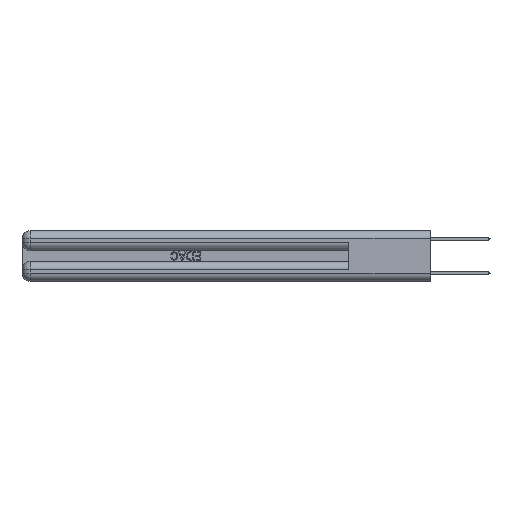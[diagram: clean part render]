
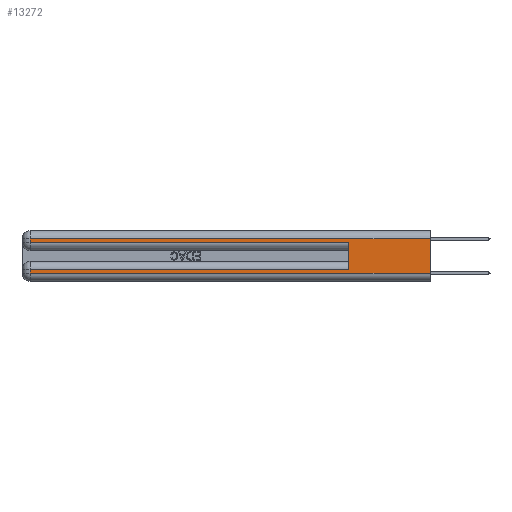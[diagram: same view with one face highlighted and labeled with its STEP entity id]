
A CAD part, left-side view. The second image highlights one B-rep face of the part: STEP entity #13272.
In plain terms, the highlighted planar face has unit normal (-1, 0, 0).
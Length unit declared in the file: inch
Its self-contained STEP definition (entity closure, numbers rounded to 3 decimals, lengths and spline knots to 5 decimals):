
#130 = CARTESIAN_POINT ( 'NONE',  ( 0., 0., 0.37 ) ) ;
#244 = DIRECTION ( 'NONE',  ( 0., 0., -1. ) ) ;
#490 = DIRECTION ( 'NONE',  ( 0., -1., 0. ) ) ;
#535 = CARTESIAN_POINT ( 'NONE',  ( 0., 0., 0.37 ) ) ;
#685 = AXIS2_PLACEMENT_3D ( 'NONE', #130, #22805, #11652 ) ;
#1635 = CARTESIAN_POINT ( 'NONE',  ( 0., 0.6, 0.085 ) ) ;
#1852 = ORIENTED_EDGE ( 'NONE', *, *, #2082, .T. ) ;
#2082 = EDGE_CURVE ( 'NONE', #6087, #33035, #23856, .T. ) ;
#2722 = CARTESIAN_POINT ( 'NONE',  ( 0., 0., 0.06 ) ) ;
#3221 = ORIENTED_EDGE ( 'NONE', *, *, #21603, .F. ) ;
#3281 = LINE ( 'NONE', #2722, #4337 ) ;
#3654 = EDGE_CURVE ( 'NONE', #15670, #11428, #26232, .T. ) ;
#4158 = CARTESIAN_POINT ( 'NONE',  ( 0., 0., 0.06 ) ) ;
#4337 = VECTOR ( 'NONE', #490, 39.37008 ) ;
#5796 = VECTOR ( 'NONE', #18809, 39.37008 ) ;
#5928 = CARTESIAN_POINT ( 'NONE',  ( 0., 2.94, 0.285 ) ) ;
#5946 = EDGE_CURVE ( 'NONE', #33035, #25880, #15562, .T. ) ;
#6087 = VERTEX_POINT ( 'NONE', #1635 ) ;
#6418 = EDGE_CURVE ( 'NONE', #6087, #16569, #23719, .T. ) ;
#6473 = CARTESIAN_POINT ( 'NONE',  ( 0., 2.94, 0.37 ) ) ;
#7280 = CARTESIAN_POINT ( 'NONE',  ( 0., 0., 0.285 ) ) ;
#7645 = ORIENTED_EDGE ( 'NONE', *, *, #17243, .T. ) ;
#8896 = VECTOR ( 'NONE', #15310, 39.37008 ) ;
#9559 = LINE ( 'NONE', #29604, #14736 ) ;
#10016 = ORIENTED_EDGE ( 'NONE', *, *, #5946, .T. ) ;
#11428 = VERTEX_POINT ( 'NONE', #5928 ) ;
#11595 = VECTOR ( 'NONE', #20779, 39.37008 ) ;
#11652 = DIRECTION ( 'NONE',  ( 0., 0., -1. ) ) ;
#12720 = DIRECTION ( 'NONE',  ( 0., 1., 0. ) ) ;
#13272 = ADVANCED_FACE ( 'NONE', ( #22987 ), #25935, .F. ) ;
#14736 = VECTOR ( 'NONE', #12720, 39.37008 ) ;
#15310 = DIRECTION ( 'NONE',  ( 0., 1., 0. ) ) ;
#15562 = LINE ( 'NONE', #6473, #11595 ) ;
#15670 = VERTEX_POINT ( 'NONE', #23554 ) ;
#15730 = CARTESIAN_POINT ( 'NONE',  ( 0., 2.94, 0.06 ) ) ;
#16569 = VERTEX_POINT ( 'NONE', #35705 ) ;
#17243 = EDGE_CURVE ( 'NONE', #25880, #35130, #3281, .T. ) ;
#17731 = VERTEX_POINT ( 'NONE', #25338 ) ;
#18809 = DIRECTION ( 'NONE',  ( 0., -1., 0. ) ) ;
#20038 = ORIENTED_EDGE ( 'NONE', *, *, #26740, .T. ) ;
#20779 = DIRECTION ( 'NONE',  ( 0., 0., -1. ) ) ;
#21052 = LINE ( 'NONE', #7280, #5796 ) ;
#21603 = EDGE_CURVE ( 'NONE', #17731, #35130, #34700, .T. ) ;
#22805 = DIRECTION ( 'NONE',  ( 1., 0., 0. ) ) ;
#22808 = ORIENTED_EDGE ( 'NONE', *, *, #27815, .T. ) ;
#22987 = FACE_OUTER_BOUND ( 'NONE', #29051, .T. ) ;
#23554 = CARTESIAN_POINT ( 'NONE',  ( 0., 2.94, 0.31 ) ) ;
#23719 = LINE ( 'NONE', #30005, #33558 ) ;
#23856 = LINE ( 'NONE', #26453, #8896 ) ;
#24526 = VECTOR ( 'NONE', #244, 39.37008 ) ;
#25186 = ORIENTED_EDGE ( 'NONE', *, *, #6418, .F. ) ;
#25338 = CARTESIAN_POINT ( 'NONE',  ( 0., 0., 0.31 ) ) ;
#25880 = VERTEX_POINT ( 'NONE', #15730 ) ;
#25935 = PLANE ( 'NONE',  #685 ) ;
#26232 = LINE ( 'NONE', #28287, #24526 ) ;
#26453 = CARTESIAN_POINT ( 'NONE',  ( 0., 0., 0.085 ) ) ;
#26740 = EDGE_CURVE ( 'NONE', #11428, #16569, #21052, .T. ) ;
#27815 = EDGE_CURVE ( 'NONE', #17731, #15670, #9559, .T. ) ;
#28287 = CARTESIAN_POINT ( 'NONE',  ( 0., 2.94, 0.37 ) ) ;
#29051 = EDGE_LOOP ( 'NONE', ( #3221, #22808, #35507, #20038, #25186, #1852, #10016, #7645 ) ) ;
#29604 = CARTESIAN_POINT ( 'NONE',  ( 0., 0., 0.31 ) ) ;
#30005 = CARTESIAN_POINT ( 'NONE',  ( 0., 0.6, 0.145 ) ) ;
#33035 = VERTEX_POINT ( 'NONE', #35373 ) ;
#33558 = VECTOR ( 'NONE', #35404, 39.37008 ) ;
#34150 = DIRECTION ( 'NONE',  ( 0., 0., -1. ) ) ;
#34700 = LINE ( 'NONE', #535, #34803 ) ;
#34803 = VECTOR ( 'NONE', #34150, 39.37008 ) ;
#35130 = VERTEX_POINT ( 'NONE', #4158 ) ;
#35373 = CARTESIAN_POINT ( 'NONE',  ( 0., 2.94, 0.085 ) ) ;
#35404 = DIRECTION ( 'NONE',  ( 0., 0., 1. ) ) ;
#35507 = ORIENTED_EDGE ( 'NONE', *, *, #3654, .T. ) ;
#35705 = CARTESIAN_POINT ( 'NONE',  ( 0., 0.6, 0.285 ) ) ;
